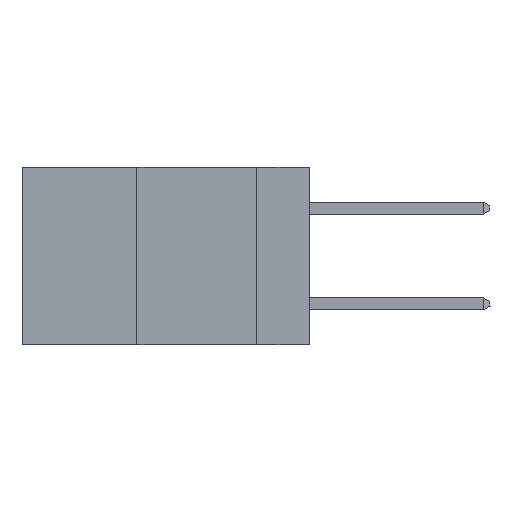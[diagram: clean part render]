
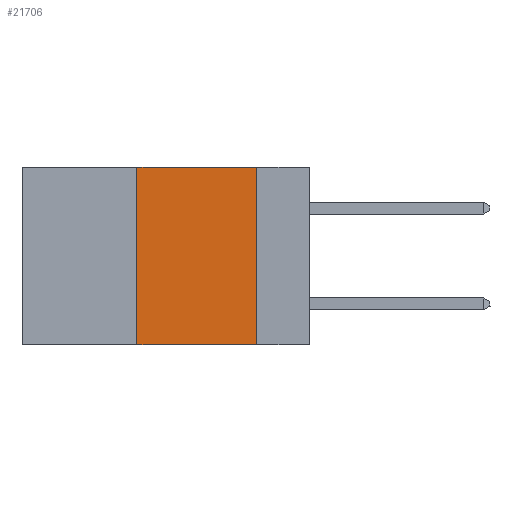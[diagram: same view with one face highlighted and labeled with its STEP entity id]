
A CAD part, left-side view. The second image highlights one B-rep face of the part: STEP entity #21706.
In plain terms, the highlighted planar face has unit normal (-1, 0, 0).
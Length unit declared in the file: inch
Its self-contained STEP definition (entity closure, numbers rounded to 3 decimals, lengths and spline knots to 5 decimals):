
#1405 = EDGE_CURVE ( 'NONE', #16644, #3941, #18810, .T. ) ;
#2182 = DIRECTION ( 'NONE',  ( 0., 0., 1. ) ) ;
#2689 = CARTESIAN_POINT ( 'NONE',  ( 0., 0.36, 0. ) ) ;
#2786 = ORIENTED_EDGE ( 'NONE', *, *, #25706, .F. ) ;
#3086 = VECTOR ( 'NONE', #2182, 39.37008 ) ;
#3137 = CARTESIAN_POINT ( 'NONE',  ( 0., 0.36, 0. ) ) ;
#3264 = DIRECTION ( 'NONE',  ( 1., 0., 0. ) ) ;
#3644 = CARTESIAN_POINT ( 'NONE',  ( 0., 0.11, 0. ) ) ;
#3941 = VERTEX_POINT ( 'NONE', #3137 ) ;
#3958 = FACE_OUTER_BOUND ( 'NONE', #15270, .T. ) ;
#4817 = CARTESIAN_POINT ( 'NONE',  ( 0., 0.11, 0. ) ) ;
#6019 = ORIENTED_EDGE ( 'NONE', *, *, #20549, .T. ) ;
#6053 = CARTESIAN_POINT ( 'NONE',  ( 0., 0.6, 0. ) ) ;
#7944 = VECTOR ( 'NONE', #11440, 39.37008 ) ;
#9437 = DIRECTION ( 'NONE',  ( 0., -1., 0. ) ) ;
#10298 = VECTOR ( 'NONE', #9437, 39.37008 ) ;
#11440 = DIRECTION ( 'NONE',  ( 0., 0., -1. ) ) ;
#11732 = CARTESIAN_POINT ( 'NONE',  ( 0., 0.6, 0. ) ) ;
#12855 = ORIENTED_EDGE ( 'NONE', *, *, #1405, .F. ) ;
#14092 = ORIENTED_EDGE ( 'NONE', *, *, #18712, .F. ) ;
#15270 = EDGE_LOOP ( 'NONE', ( #14092, #2786, #12855, #6019 ) ) ;
#15723 = DIRECTION ( 'NONE',  ( 0., -1., 0. ) ) ;
#15803 = LINE ( 'NONE', #3644, #7944 ) ;
#16644 = VERTEX_POINT ( 'NONE', #19634 ) ;
#17321 = PLANE ( 'NONE',  #17898 ) ;
#17560 = VECTOR ( 'NONE', #15723, 39.37008 ) ;
#17898 = AXIS2_PLACEMENT_3D ( 'NONE', #6053, #3264, #22392 ) ;
#18191 = LINE ( 'NONE', #11732, #17560 ) ;
#18542 = CARTESIAN_POINT ( 'NONE',  ( 0., 0.11, -0.37 ) ) ;
#18712 = EDGE_CURVE ( 'NONE', #21523, #21068, #15803, .T. ) ;
#18810 = LINE ( 'NONE', #2689, #3086 ) ;
#19634 = CARTESIAN_POINT ( 'NONE',  ( 0., 0.36, -0.37 ) ) ;
#20549 = EDGE_CURVE ( 'NONE', #16644, #21068, #22831, .T. ) ;
#21068 = VERTEX_POINT ( 'NONE', #18542 ) ;
#21523 = VERTEX_POINT ( 'NONE', #4817 ) ;
#21706 = ADVANCED_FACE ( 'NONE', ( #3958 ), #17321, .F. ) ;
#22392 = DIRECTION ( 'NONE',  ( 0., 0., -1. ) ) ;
#22831 = LINE ( 'NONE', #23220, #10298 ) ;
#23220 = CARTESIAN_POINT ( 'NONE',  ( 0., 0.6, -0.37 ) ) ;
#25706 = EDGE_CURVE ( 'NONE', #3941, #21523, #18191, .T. ) ;
